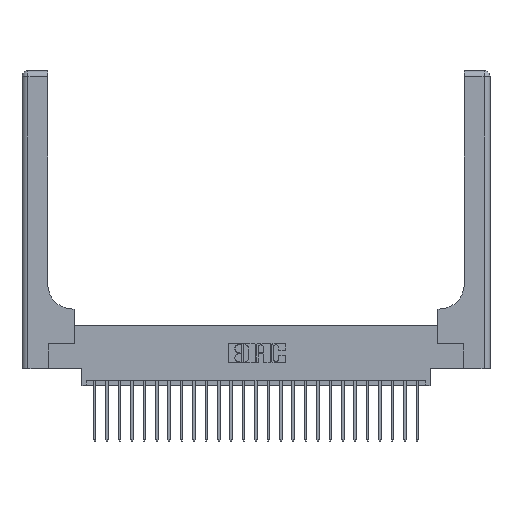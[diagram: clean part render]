
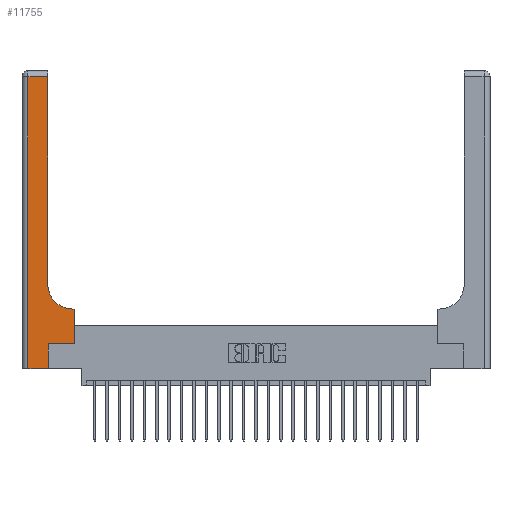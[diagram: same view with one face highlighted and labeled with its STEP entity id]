
A CAD part, top view. The second image highlights one B-rep face of the part: STEP entity #11755.
In plain terms, the highlighted planar face has unit normal (0, 0, 1).
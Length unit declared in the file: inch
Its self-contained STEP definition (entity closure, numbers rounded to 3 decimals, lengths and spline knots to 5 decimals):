
#197 = VECTOR ( 'NONE', #12969, 39.37008 ) ;
#307 = LINE ( 'NONE', #23714, #3536 ) ;
#362 = VERTEX_POINT ( 'NONE', #10499 ) ;
#572 = VECTOR ( 'NONE', #1948, 39.37008 ) ;
#689 = CIRCLE ( 'NONE', #8923, 0.25 ) ;
#809 = DIRECTION ( 'NONE',  ( 0., 0., -1. ) ) ;
#1006 = EDGE_CURVE ( 'NONE', #9976, #13815, #21879, .T. ) ;
#1348 = ORIENTED_EDGE ( 'NONE', *, *, #2914, .T. ) ;
#1568 = VERTEX_POINT ( 'NONE', #10373 ) ;
#1948 = DIRECTION ( 'NONE',  ( -1., 0., 0. ) ) ;
#2138 = DIRECTION ( 'NONE',  ( -1., 0., 0. ) ) ;
#2914 = EDGE_CURVE ( 'NONE', #10034, #9976, #15948, .T. ) ;
#3259 = EDGE_CURVE ( 'NONE', #7100, #3690, #5243, .T. ) ;
#3536 = VECTOR ( 'NONE', #4290, 39.37008 ) ;
#3690 = VERTEX_POINT ( 'NONE', #19079 ) ;
#4290 = DIRECTION ( 'NONE',  ( 0., 1., 0. ) ) ;
#4564 = LINE ( 'NONE', #21934, #25315 ) ;
#4801 = LINE ( 'NONE', #22162, #13761 ) ;
#4934 = AXIS2_PLACEMENT_3D ( 'NONE', #14434, #15758, #2138 ) ;
#5243 = LINE ( 'NONE', #20803, #197 ) ;
#5710 = ORIENTED_EDGE ( 'NONE', *, *, #1006, .T. ) ;
#7100 = VERTEX_POINT ( 'NONE', #8774 ) ;
#8669 = DIRECTION ( 'NONE',  ( 1., 0., 0. ) ) ;
#8774 = CARTESIAN_POINT ( 'NONE',  ( 0.528, 0.25, 0.37 ) ) ;
#8923 = AXIS2_PLACEMENT_3D ( 'NONE', #18432, #809, #8669 ) ;
#9276 = LINE ( 'NONE', #19421, #572 ) ;
#9378 = EDGE_CURVE ( 'NONE', #3690, #9928, #9276, .T. ) ;
#9555 = DIRECTION ( 'NONE',  ( -1., 0., 0. ) ) ;
#9928 = VERTEX_POINT ( 'NONE', #18560 ) ;
#9938 = EDGE_CURVE ( 'NONE', #13815, #362, #4801, .T. ) ;
#9976 = VERTEX_POINT ( 'NONE', #10723 ) ;
#10034 = VERTEX_POINT ( 'NONE', #12656 ) ;
#10373 = CARTESIAN_POINT ( 'NONE',  ( 0.265, 0.25, 0.37 ) ) ;
#10499 = CARTESIAN_POINT ( 'NONE',  ( 0.06, 0., 0.37 ) ) ;
#10723 = CARTESIAN_POINT ( 'NONE',  ( 0.26, 2.94, 0.37 ) ) ;
#11239 = ORIENTED_EDGE ( 'NONE', *, *, #3259, .T. ) ;
#11275 = ORIENTED_EDGE ( 'NONE', *, *, #16684, .T. ) ;
#11755 = ADVANCED_FACE ( 'NONE', ( #20336 ), #19739, .F. ) ;
#11923 = ORIENTED_EDGE ( 'NONE', *, *, #17543, .T. ) ;
#12656 = CARTESIAN_POINT ( 'NONE',  ( 0.26, 0.85, 0.37 ) ) ;
#12969 = DIRECTION ( 'NONE',  ( 0., 1., 0. ) ) ;
#13231 = CARTESIAN_POINT ( 'NONE',  ( 0.06, 2.94, 0.37 ) ) ;
#13761 = VECTOR ( 'NONE', #18177, 39.37008 ) ;
#13815 = VERTEX_POINT ( 'NONE', #13231 ) ;
#14434 = CARTESIAN_POINT ( 'NONE',  ( 0., 3., 0.37 ) ) ;
#15535 = ORIENTED_EDGE ( 'NONE', *, *, #9378, .T. ) ;
#15719 = ORIENTED_EDGE ( 'NONE', *, *, #16243, .T. ) ;
#15758 = DIRECTION ( 'NONE',  ( 0., 0., -1. ) ) ;
#15948 = LINE ( 'NONE', #19796, #23144 ) ;
#16024 = DIRECTION ( 'NONE',  ( 1., 0., 0. ) ) ;
#16230 = VECTOR ( 'NONE', #9555, 39.37008 ) ;
#16243 = EDGE_CURVE ( 'NONE', #1568, #7100, #4564, .T. ) ;
#16684 = EDGE_CURVE ( 'NONE', #17726, #1568, #307, .T. ) ;
#17543 = EDGE_CURVE ( 'NONE', #362, #17726, #21969, .T. ) ;
#17726 = VERTEX_POINT ( 'NONE', #18490 ) ;
#17990 = DIRECTION ( 'NONE',  ( 1., 0., 0. ) ) ;
#18090 = ORIENTED_EDGE ( 'NONE', *, *, #19853, .T. ) ;
#18177 = DIRECTION ( 'NONE',  ( 0., -1., 0. ) ) ;
#18432 = CARTESIAN_POINT ( 'NONE',  ( 0.51, 0.85, 0.37 ) ) ;
#18490 = CARTESIAN_POINT ( 'NONE',  ( 0.265, 0., 0.37 ) ) ;
#18560 = CARTESIAN_POINT ( 'NONE',  ( 0.51, 0.6, 0.37 ) ) ;
#19079 = CARTESIAN_POINT ( 'NONE',  ( 0.528, 0.6, 0.37 ) ) ;
#19421 = CARTESIAN_POINT ( 'NONE',  ( 0.26, 0.6, 0.37 ) ) ;
#19739 = PLANE ( 'NONE',  #4934 ) ;
#19796 = CARTESIAN_POINT ( 'NONE',  ( 0.26, 3., 0.37 ) ) ;
#19853 = EDGE_CURVE ( 'NONE', #9928, #10034, #689, .T. ) ;
#20336 = FACE_OUTER_BOUND ( 'NONE', #22667, .T. ) ;
#20803 = CARTESIAN_POINT ( 'NONE',  ( 0.528, 0.25, 0.37 ) ) ;
#21879 = LINE ( 'NONE', #25250, #16230 ) ;
#21934 = CARTESIAN_POINT ( 'NONE',  ( 0.265, 0.25, 0.37 ) ) ;
#21969 = LINE ( 'NONE', #23388, #25351 ) ;
#22162 = CARTESIAN_POINT ( 'NONE',  ( 0.06, 3., 0.37 ) ) ;
#22667 = EDGE_LOOP ( 'NONE', ( #1348, #5710, #25103, #11923, #11275, #15719, #11239, #15535, #18090 ) ) ;
#23144 = VECTOR ( 'NONE', #23666, 39.37008 ) ;
#23388 = CARTESIAN_POINT ( 'NONE',  ( 0., 0., 0.37 ) ) ;
#23666 = DIRECTION ( 'NONE',  ( 0., 1., 0. ) ) ;
#23714 = CARTESIAN_POINT ( 'NONE',  ( 0.265, 0., 0.37 ) ) ;
#25103 = ORIENTED_EDGE ( 'NONE', *, *, #9938, .T. ) ;
#25250 = CARTESIAN_POINT ( 'NONE',  ( 0., 2.94, 0.37 ) ) ;
#25315 = VECTOR ( 'NONE', #16024, 39.37008 ) ;
#25351 = VECTOR ( 'NONE', #17990, 39.37008 ) ;
